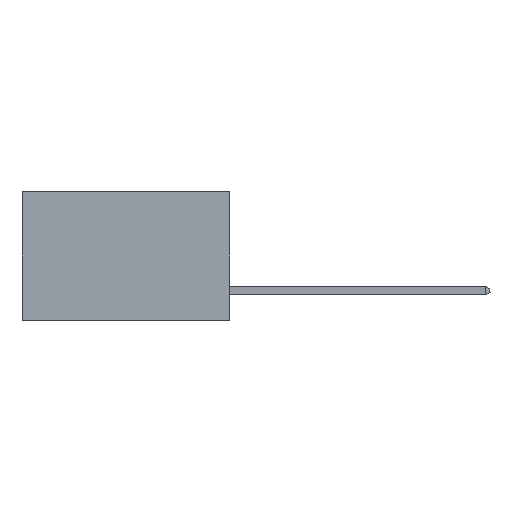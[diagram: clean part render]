
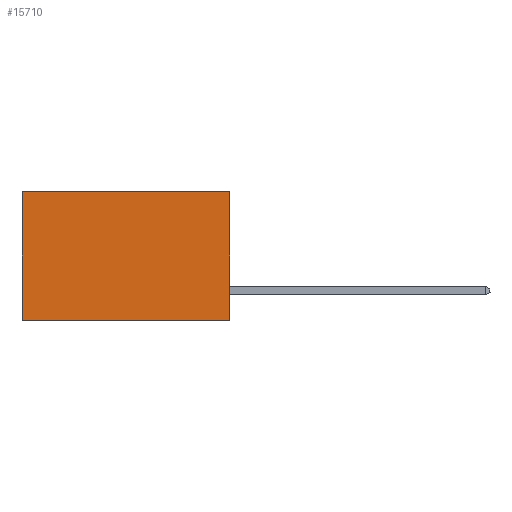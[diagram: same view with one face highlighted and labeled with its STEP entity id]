
A CAD part, left-side view. The second image highlights one B-rep face of the part: STEP entity #15710.
In plain terms, the highlighted planar face has unit normal (-1, 0, 0).
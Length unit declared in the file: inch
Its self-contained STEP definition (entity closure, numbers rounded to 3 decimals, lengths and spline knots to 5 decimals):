
#89 = CARTESIAN_POINT ( 'NONE',  ( 0.298, 0., 0. ) ) ;
#304 = LINE ( 'NONE', #6940, #6984 ) ;
#630 = EDGE_CURVE ( 'NONE', #6755, #9750, #9060, .T. ) ;
#916 = ORIENTED_EDGE ( 'NONE', *, *, #9969, .F. ) ;
#1097 = VERTEX_POINT ( 'NONE', #12172 ) ;
#1172 = LINE ( 'NONE', #89, #1979 ) ;
#1465 = PLANE ( 'NONE',  #10836 ) ;
#1979 = VECTOR ( 'NONE', #4008, 39.37008 ) ;
#3125 = FACE_OUTER_BOUND ( 'NONE', #14848, .T. ) ;
#3234 = VERTEX_POINT ( 'NONE', #3294 ) ;
#3294 = CARTESIAN_POINT ( 'NONE',  ( 0.298, 0.6, -0.37 ) ) ;
#4008 = DIRECTION ( 'NONE',  ( 0., 0., -1. ) ) ;
#5495 = VECTOR ( 'NONE', #8973, 39.37008 ) ;
#6753 = CARTESIAN_POINT ( 'NONE',  ( 0.298, 0.6, 0. ) ) ;
#6755 = VERTEX_POINT ( 'NONE', #10453 ) ;
#6768 = EDGE_CURVE ( 'NONE', #6755, #1097, #1172, .T. ) ;
#6940 = CARTESIAN_POINT ( 'NONE',  ( 0.298, 0., -0.37 ) ) ;
#6984 = VECTOR ( 'NONE', #13478, 39.37008 ) ;
#7411 = ORIENTED_EDGE ( 'NONE', *, *, #13973, .T. ) ;
#7547 = DIRECTION ( 'NONE',  ( 0., 1., 0. ) ) ;
#7955 = DIRECTION ( 'NONE',  ( 1., 0., 0. ) ) ;
#8908 = LINE ( 'NONE', #15368, #5495 ) ;
#8973 = DIRECTION ( 'NONE',  ( 0., 0., -1. ) ) ;
#9060 = LINE ( 'NONE', #15365, #13125 ) ;
#9317 = DIRECTION ( 'NONE',  ( 0., 0., -1. ) ) ;
#9750 = VERTEX_POINT ( 'NONE', #6753 ) ;
#9969 = EDGE_CURVE ( 'NONE', #1097, #3234, #304, .T. ) ;
#10453 = CARTESIAN_POINT ( 'NONE',  ( 0.298, 0., 0. ) ) ;
#10836 = AXIS2_PLACEMENT_3D ( 'NONE', #11803, #7955, #9317 ) ;
#11803 = CARTESIAN_POINT ( 'NONE',  ( 0.298, 0., 0. ) ) ;
#12172 = CARTESIAN_POINT ( 'NONE',  ( 0.298, 0., -0.37 ) ) ;
#13125 = VECTOR ( 'NONE', #7547, 39.37008 ) ;
#13478 = DIRECTION ( 'NONE',  ( 0., 1., 0. ) ) ;
#13973 = EDGE_CURVE ( 'NONE', #9750, #3234, #8908, .T. ) ;
#14848 = EDGE_LOOP ( 'NONE', ( #7411, #916, #15345, #14948 ) ) ;
#14948 = ORIENTED_EDGE ( 'NONE', *, *, #630, .T. ) ;
#15345 = ORIENTED_EDGE ( 'NONE', *, *, #6768, .F. ) ;
#15365 = CARTESIAN_POINT ( 'NONE',  ( 0.298, 0., 0. ) ) ;
#15368 = CARTESIAN_POINT ( 'NONE',  ( 0.298, 0.6, 0. ) ) ;
#15710 = ADVANCED_FACE ( 'NONE', ( #3125 ), #1465, .F. ) ;
